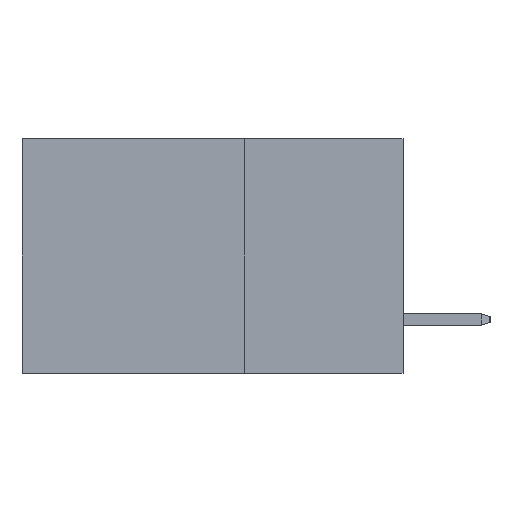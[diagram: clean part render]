
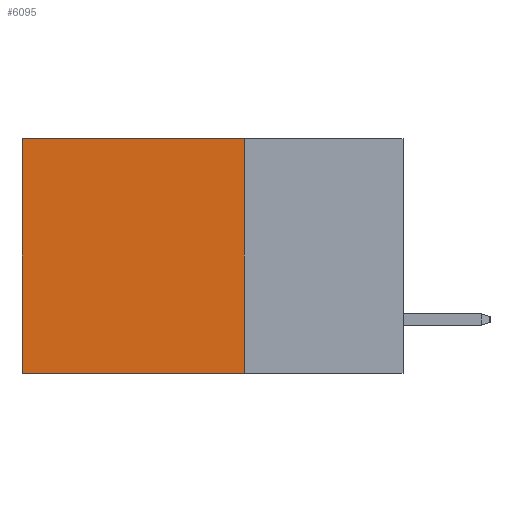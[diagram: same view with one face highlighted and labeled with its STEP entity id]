
A CAD part, left-side view. The second image highlights one B-rep face of the part: STEP entity #6095.
In plain terms, the highlighted planar face has unit normal (-1, 0, 0).
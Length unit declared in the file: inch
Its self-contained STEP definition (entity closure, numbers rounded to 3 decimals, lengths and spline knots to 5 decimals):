
#19 = DIRECTION ( 'NONE',  ( 0., 1., 0. ) ) ;
#235 = EDGE_CURVE ( 'NONE', #8563, #6588, #9696, .T. ) ;
#340 = CARTESIAN_POINT ( 'NONE',  ( 0.2875, 0.25, 0. ) ) ;
#934 = CARTESIAN_POINT ( 'NONE',  ( 0.2875, 0.6, 0. ) ) ;
#1037 = FACE_OUTER_BOUND ( 'NONE', #6575, .T. ) ;
#1928 = EDGE_CURVE ( 'NONE', #11888, #6144, #6697, .T. ) ;
#2405 = ORIENTED_EDGE ( 'NONE', *, *, #5685, .T. ) ;
#2973 = ORIENTED_EDGE ( 'NONE', *, *, #235, .T. ) ;
#2993 = CARTESIAN_POINT ( 'NONE',  ( 0.2875, 0.25, 0. ) ) ;
#3303 = LINE ( 'NONE', #340, #9501 ) ;
#3312 = CARTESIAN_POINT ( 'NONE',  ( 0.2875, 0.25, -0.37 ) ) ;
#5254 = VECTOR ( 'NONE', #11825, 39.37008 ) ;
#5414 = PLANE ( 'NONE',  #12197 ) ;
#5685 = EDGE_CURVE ( 'NONE', #11888, #8563, #3303, .T. ) ;
#6095 = ADVANCED_FACE ( 'NONE', ( #1037 ), #5414, .F. ) ;
#6144 = VERTEX_POINT ( 'NONE', #3312 ) ;
#6428 = DIRECTION ( 'NONE',  ( 0., 0., -1. ) ) ;
#6549 = DIRECTION ( 'NONE',  ( 0., 1., 0. ) ) ;
#6575 = EDGE_LOOP ( 'NONE', ( #2973, #10749, #13582, #2405 ) ) ;
#6588 = VERTEX_POINT ( 'NONE', #10808 ) ;
#6697 = LINE ( 'NONE', #8938, #11980 ) ;
#6836 = DIRECTION ( 'NONE',  ( 0., 0., -1. ) ) ;
#8414 = EDGE_CURVE ( 'NONE', #6144, #6588, #13684, .T. ) ;
#8563 = VERTEX_POINT ( 'NONE', #13194 ) ;
#8640 = VECTOR ( 'NONE', #19, 39.37008 ) ;
#8938 = CARTESIAN_POINT ( 'NONE',  ( 0.2875, 0.25, 0. ) ) ;
#9501 = VECTOR ( 'NONE', #6549, 39.37008 ) ;
#9696 = LINE ( 'NONE', #934, #5254 ) ;
#10686 = DIRECTION ( 'NONE',  ( 1., 0., 0. ) ) ;
#10749 = ORIENTED_EDGE ( 'NONE', *, *, #8414, .F. ) ;
#10808 = CARTESIAN_POINT ( 'NONE',  ( 0.2875, 0.6, -0.37 ) ) ;
#11677 = CARTESIAN_POINT ( 'NONE',  ( 0.2875, 0.25, -0.37 ) ) ;
#11825 = DIRECTION ( 'NONE',  ( 0., 0., -1. ) ) ;
#11888 = VERTEX_POINT ( 'NONE', #2993 ) ;
#11980 = VECTOR ( 'NONE', #6836, 39.37008 ) ;
#12197 = AXIS2_PLACEMENT_3D ( 'NONE', #12856, #10686, #6428 ) ;
#12856 = CARTESIAN_POINT ( 'NONE',  ( 0.2875, 0.25, 0. ) ) ;
#13194 = CARTESIAN_POINT ( 'NONE',  ( 0.2875, 0.6, 0. ) ) ;
#13582 = ORIENTED_EDGE ( 'NONE', *, *, #1928, .F. ) ;
#13684 = LINE ( 'NONE', #11677, #8640 ) ;
